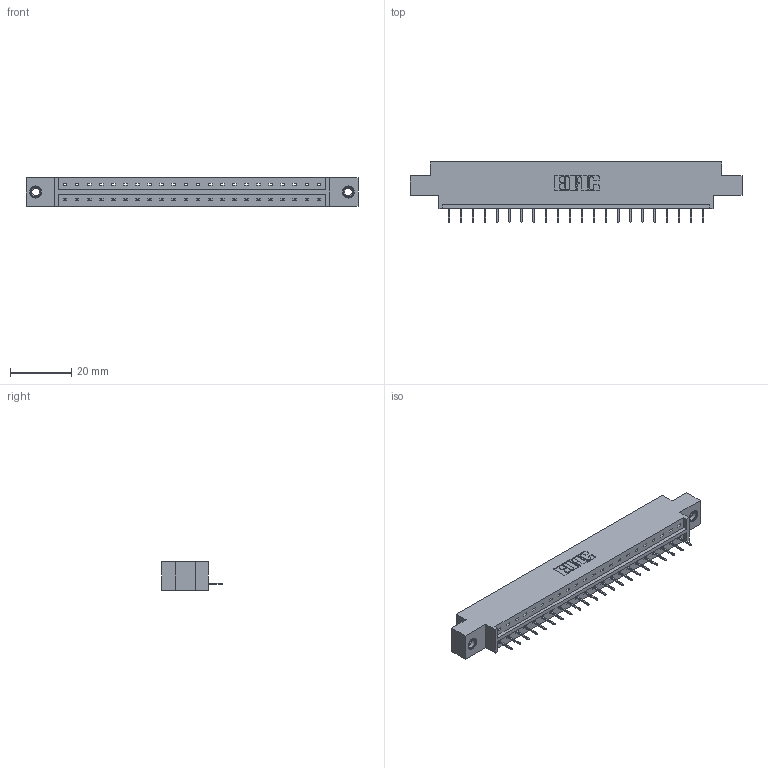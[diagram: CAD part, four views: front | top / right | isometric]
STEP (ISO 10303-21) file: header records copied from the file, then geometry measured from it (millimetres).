
FILE_DESCRIPTION (( 'STEP AP203' ), '1' );
FILE_NAME ('833-022-524-607.STEP', '2020-06-01T16:43:26', ( '' ), ( '' ), 'SwSTEP 2.0', 'SolidWorks 2020', '' );
FILE_SCHEMA (( 'CONFIG_CONTROL_DESIGN' ));
Length unit declared in the file: inch
Products named in the file (4): 833-022-524-607; 833 Part_Offset - .156 Dia - TI; 345-250-001_345-250-005-103; 345-292-001_345-293-124
Assembly tree (25 placements, depth 2):
  833-022-524-607
    833 Part_Offset - .156 Dia - TI
    345-292-001_345-293-124  x22
    345-250-001_345-250-005-103  x2
Bounding box: 108.71 x 19.69 x 9.4 mm (x, y, z)
Volume: 10439.3 mm3; surface area: 11101.1 mm2
Topology: 25 solids, 25 shells, 1542 faces, 4419 edges, 2850 vertices
Faces by surface type: plane 1162, cylinder 364, cone 12, torus 4
Entity records: 17428 total; most frequent: CARTESIAN_POINT 2991, ORIENTED_EDGE 2942, DIRECTION 2597, EDGE_CURVE 1471, LINE 1327, VECTOR 1327, VERTEX_POINT 972, AXIS2_PLACEMENT_3D 635
